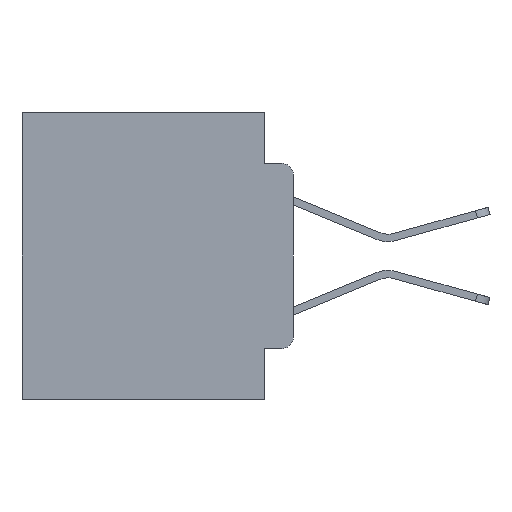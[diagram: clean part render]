
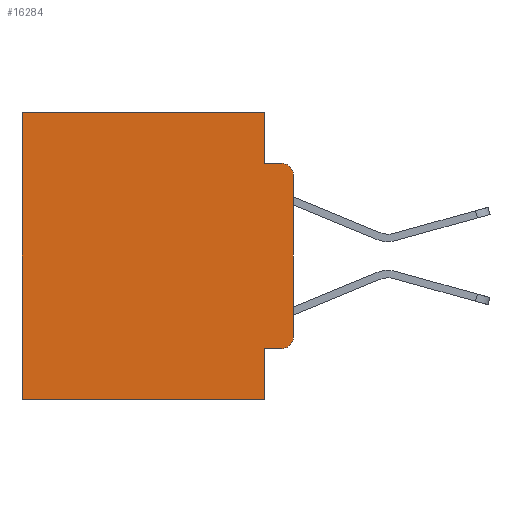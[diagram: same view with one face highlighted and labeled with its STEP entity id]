
A CAD part, left-side view. The second image highlights one B-rep face of the part: STEP entity #16284.
In plain terms, the highlighted planar face has unit normal (-1, 0, 0).
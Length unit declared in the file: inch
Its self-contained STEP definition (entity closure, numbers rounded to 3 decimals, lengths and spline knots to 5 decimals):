
#377 = VERTEX_POINT ( 'NONE', #24490 ) ;
#764 = DIRECTION ( 'NONE',  ( 1., 0., 0. ) ) ;
#787 = VERTEX_POINT ( 'NONE', #21621 ) ;
#1449 = VECTOR ( 'NONE', #26264, 39.37008 ) ;
#1515 = ORIENTED_EDGE ( 'NONE', *, *, #20760, .F. ) ;
#2415 = CARTESIAN_POINT ( 'NONE',  ( 0.298, 0.473, -0.5 ) ) ;
#2555 = CARTESIAN_POINT ( 'NONE',  ( 0.298, 0., -0.1085 ) ) ;
#3775 = EDGE_CURVE ( 'NONE', #22813, #787, #24047, .T. ) ;
#3911 = VERTEX_POINT ( 'NONE', #21743 ) ;
#4218 = CARTESIAN_POINT ( 'NONE',  ( 0.298, 0.02, -0.4115 ) ) ;
#4465 = VERTEX_POINT ( 'NONE', #2415 ) ;
#5185 = EDGE_LOOP ( 'NONE', ( #23332, #24017, #21955, #1515, #24718, #18160, #18865, #15977, #27734, #7937 ) ) ;
#5523 = LINE ( 'NONE', #9151, #28487 ) ;
#5997 = CARTESIAN_POINT ( 'NONE',  ( 0.298, 0.051, -0.0885 ) ) ;
#6081 = CARTESIAN_POINT ( 'NONE',  ( 0.298, 0.051, -0.0885 ) ) ;
#6644 = EDGE_CURVE ( 'NONE', #3911, #4465, #10172, .T. ) ;
#7156 = CARTESIAN_POINT ( 'NONE',  ( 0.298, 0.051, 0. ) ) ;
#7584 = LINE ( 'NONE', #10710, #1449 ) ;
#7937 = ORIENTED_EDGE ( 'NONE', *, *, #13281, .T. ) ;
#8455 = DIRECTION ( 'NONE',  ( 0., 1., 0. ) ) ;
#8628 = CARTESIAN_POINT ( 'NONE',  ( 0.298, 0.02, -0.1085 ) ) ;
#8858 = CARTESIAN_POINT ( 'NONE',  ( 0.298, 0.02, -0.3915 ) ) ;
#9151 = CARTESIAN_POINT ( 'NONE',  ( 0.298, 0.051, 0. ) ) ;
#9484 = LINE ( 'NONE', #5997, #14748 ) ;
#9566 = CIRCLE ( 'NONE', #15787, 0.02 ) ;
#10172 = LINE ( 'NONE', #14365, #20664 ) ;
#10189 = FACE_OUTER_BOUND ( 'NONE', #5185, .T. ) ;
#10710 = CARTESIAN_POINT ( 'NONE',  ( 0.298, 0., 0. ) ) ;
#10865 = DIRECTION ( 'NONE',  ( 0., 0., -1. ) ) ;
#11011 = LINE ( 'NONE', #12126, #16289 ) ;
#11099 = DIRECTION ( 'NONE',  ( 0., 0., -1. ) ) ;
#11414 = DIRECTION ( 'NONE',  ( 0., 0., -1. ) ) ;
#11675 = LINE ( 'NONE', #7156, #16938 ) ;
#12126 = CARTESIAN_POINT ( 'NONE',  ( 0.298, 0.473, 0. ) ) ;
#13281 = EDGE_CURVE ( 'NONE', #24910, #14273, #24656, .T. ) ;
#13918 = DIRECTION ( 'NONE',  ( 0., 0., -1. ) ) ;
#14273 = VERTEX_POINT ( 'NONE', #21739 ) ;
#14284 = CARTESIAN_POINT ( 'NONE',  ( 0.298, 0.051, -0.4115 ) ) ;
#14347 = CARTESIAN_POINT ( 'NONE',  ( 0.298, 0., 0. ) ) ;
#14365 = CARTESIAN_POINT ( 'NONE',  ( 0.298, 0., -0.5 ) ) ;
#14388 = CARTESIAN_POINT ( 'NONE',  ( 0.298, 0., 0. ) ) ;
#14748 = VECTOR ( 'NONE', #23870, 39.37008 ) ;
#15787 = AXIS2_PLACEMENT_3D ( 'NONE', #8628, #24233, #10865 ) ;
#15903 = VERTEX_POINT ( 'NONE', #6081 ) ;
#15977 = ORIENTED_EDGE ( 'NONE', *, *, #17781, .F. ) ;
#16274 = EDGE_CURVE ( 'NONE', #377, #24910, #28585, .T. ) ;
#16284 = ADVANCED_FACE ( 'NONE', ( #10189 ), #27641, .F. ) ;
#16289 = VECTOR ( 'NONE', #25526, 39.37008 ) ;
#16550 = DIRECTION ( 'NONE',  ( 0., -1., 0. ) ) ;
#16641 = DIRECTION ( 'NONE',  ( 0., 0., -1. ) ) ;
#16938 = VECTOR ( 'NONE', #13918, 39.37008 ) ;
#17781 = EDGE_CURVE ( 'NONE', #377, #3911, #5523, .T. ) ;
#18160 = ORIENTED_EDGE ( 'NONE', *, *, #19275, .T. ) ;
#18470 = AXIS2_PLACEMENT_3D ( 'NONE', #14388, #764, #16641 ) ;
#18865 = ORIENTED_EDGE ( 'NONE', *, *, #6644, .F. ) ;
#19275 = EDGE_CURVE ( 'NONE', #787, #4465, #11011, .T. ) ;
#20664 = VECTOR ( 'NONE', #25421, 39.37008 ) ;
#20731 = VERTEX_POINT ( 'NONE', #2555 ) ;
#20760 = EDGE_CURVE ( 'NONE', #22813, #15903, #11675, .T. ) ;
#20777 = CARTESIAN_POINT ( 'NONE',  ( 0.298, 0.02, -0.0885 ) ) ;
#21621 = CARTESIAN_POINT ( 'NONE',  ( 0.298, 0.473, 0. ) ) ;
#21739 = CARTESIAN_POINT ( 'NONE',  ( 0.298, 0., -0.3915 ) ) ;
#21743 = CARTESIAN_POINT ( 'NONE',  ( 0.298, 0.051, -0.5 ) ) ;
#21955 = ORIENTED_EDGE ( 'NONE', *, *, #22247, .F. ) ;
#22247 = EDGE_CURVE ( 'NONE', #15903, #26664, #9484, .T. ) ;
#22776 = VECTOR ( 'NONE', #16550, 39.37008 ) ;
#22813 = VERTEX_POINT ( 'NONE', #25841 ) ;
#23332 = ORIENTED_EDGE ( 'NONE', *, *, #28103, .F. ) ;
#23370 = VECTOR ( 'NONE', #8455, 39.37008 ) ;
#23721 = EDGE_CURVE ( 'NONE', #20731, #26664, #9566, .T. ) ;
#23870 = DIRECTION ( 'NONE',  ( 0., -1., 0. ) ) ;
#24017 = ORIENTED_EDGE ( 'NONE', *, *, #23721, .T. ) ;
#24047 = LINE ( 'NONE', #14347, #23370 ) ;
#24233 = DIRECTION ( 'NONE',  ( -1., 0., 0. ) ) ;
#24453 = DIRECTION ( 'NONE',  ( -1., 0., 0. ) ) ;
#24490 = CARTESIAN_POINT ( 'NONE',  ( 0.298, 0.051, -0.4115 ) ) ;
#24516 = AXIS2_PLACEMENT_3D ( 'NONE', #8858, #24453, #11099 ) ;
#24656 = CIRCLE ( 'NONE', #24516, 0.02 ) ;
#24718 = ORIENTED_EDGE ( 'NONE', *, *, #3775, .T. ) ;
#24910 = VERTEX_POINT ( 'NONE', #4218 ) ;
#25421 = DIRECTION ( 'NONE',  ( 0., 1., 0. ) ) ;
#25526 = DIRECTION ( 'NONE',  ( 0., 0., -1. ) ) ;
#25841 = CARTESIAN_POINT ( 'NONE',  ( 0.298, 0.051, 0. ) ) ;
#26264 = DIRECTION ( 'NONE',  ( 0., 0., -1. ) ) ;
#26664 = VERTEX_POINT ( 'NONE', #20777 ) ;
#27641 = PLANE ( 'NONE',  #18470 ) ;
#27734 = ORIENTED_EDGE ( 'NONE', *, *, #16274, .T. ) ;
#28103 = EDGE_CURVE ( 'NONE', #20731, #14273, #7584, .T. ) ;
#28487 = VECTOR ( 'NONE', #11414, 39.37008 ) ;
#28585 = LINE ( 'NONE', #14284, #22776 ) ;
